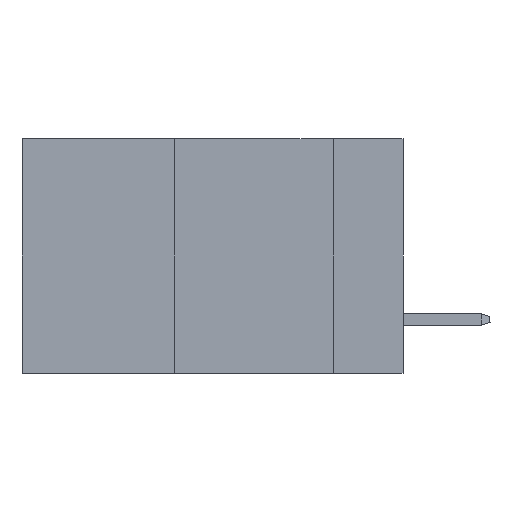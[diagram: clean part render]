
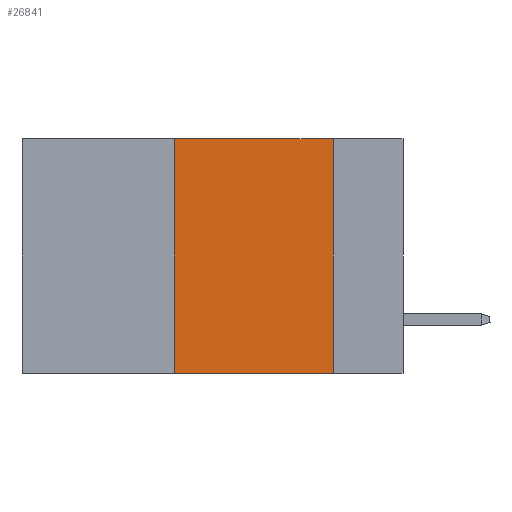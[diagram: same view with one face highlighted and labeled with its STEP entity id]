
A CAD part, left-side view. The second image highlights one B-rep face of the part: STEP entity #26841.
In plain terms, the highlighted planar face has unit normal (-1, 0, 0).
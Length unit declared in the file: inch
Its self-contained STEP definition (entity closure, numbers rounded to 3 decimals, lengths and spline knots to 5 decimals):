
#445 = DIRECTION ( 'NONE',  ( 0., -1., 0. ) ) ;
#581 = VECTOR ( 'NONE', #11583, 39.37008 ) ;
#1860 = VECTOR ( 'NONE', #445, 39.37008 ) ;
#1959 = CARTESIAN_POINT ( 'NONE',  ( 0., 0.11, -0.37 ) ) ;
#2348 = LINE ( 'NONE', #20103, #26683 ) ;
#2626 = AXIS2_PLACEMENT_3D ( 'NONE', #25155, #14076, #25440 ) ;
#2713 = CARTESIAN_POINT ( 'NONE',  ( 0., 0.6, 0. ) ) ;
#3784 = VERTEX_POINT ( 'NONE', #1959 ) ;
#9182 = DIRECTION ( 'NONE',  ( 0., 0., 1. ) ) ;
#9531 = VERTEX_POINT ( 'NONE', #13920 ) ;
#9949 = LINE ( 'NONE', #14321, #24014 ) ;
#11583 = DIRECTION ( 'NONE',  ( 0., -1., 0. ) ) ;
#11755 = FACE_OUTER_BOUND ( 'NONE', #20777, .T. ) ;
#12036 = EDGE_CURVE ( 'NONE', #9531, #3784, #26626, .T. ) ;
#13920 = CARTESIAN_POINT ( 'NONE',  ( 0., 0.36, -0.37 ) ) ;
#14076 = DIRECTION ( 'NONE',  ( 1., 0., 0. ) ) ;
#14321 = CARTESIAN_POINT ( 'NONE',  ( 0., 0.11, 0. ) ) ;
#14518 = VERTEX_POINT ( 'NONE', #24831 ) ;
#14534 = EDGE_CURVE ( 'NONE', #14518, #20545, #22649, .T. ) ;
#14786 = ORIENTED_EDGE ( 'NONE', *, *, #12036, .T. ) ;
#18561 = DIRECTION ( 'NONE',  ( 0., 0., -1. ) ) ;
#20103 = CARTESIAN_POINT ( 'NONE',  ( 0., 0.36, 0. ) ) ;
#20545 = VERTEX_POINT ( 'NONE', #23523 ) ;
#20771 = EDGE_CURVE ( 'NONE', #20545, #3784, #9949, .T. ) ;
#20777 = EDGE_LOOP ( 'NONE', ( #24281, #22370, #25607, #14786 ) ) ;
#22370 = ORIENTED_EDGE ( 'NONE', *, *, #14534, .F. ) ;
#22649 = LINE ( 'NONE', #2713, #581 ) ;
#23116 = PLANE ( 'NONE',  #2626 ) ;
#23523 = CARTESIAN_POINT ( 'NONE',  ( 0., 0.11, 0. ) ) ;
#24007 = EDGE_CURVE ( 'NONE', #9531, #14518, #2348, .T. ) ;
#24014 = VECTOR ( 'NONE', #18561, 39.37008 ) ;
#24281 = ORIENTED_EDGE ( 'NONE', *, *, #20771, .F. ) ;
#24745 = CARTESIAN_POINT ( 'NONE',  ( 0., 0.6, -0.37 ) ) ;
#24831 = CARTESIAN_POINT ( 'NONE',  ( 0., 0.36, 0. ) ) ;
#25155 = CARTESIAN_POINT ( 'NONE',  ( 0., 0.6, 0. ) ) ;
#25440 = DIRECTION ( 'NONE',  ( 0., 0., -1. ) ) ;
#25607 = ORIENTED_EDGE ( 'NONE', *, *, #24007, .F. ) ;
#26626 = LINE ( 'NONE', #24745, #1860 ) ;
#26683 = VECTOR ( 'NONE', #9182, 39.37008 ) ;
#26841 = ADVANCED_FACE ( 'NONE', ( #11755 ), #23116, .F. ) ;
